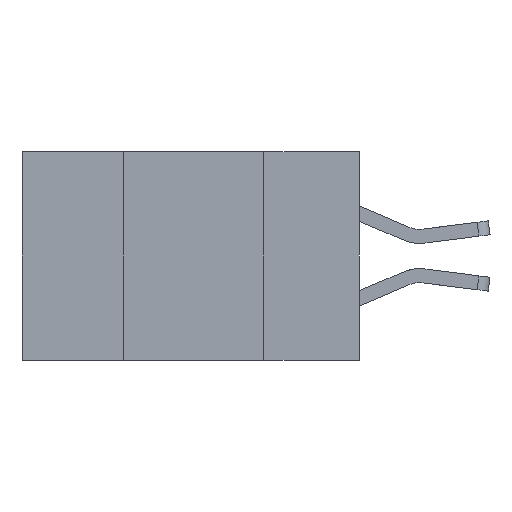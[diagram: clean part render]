
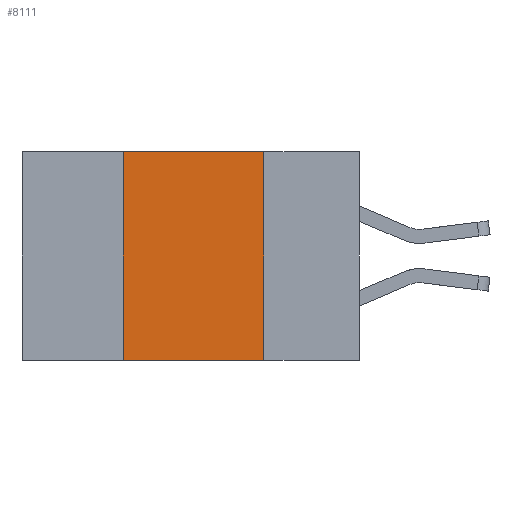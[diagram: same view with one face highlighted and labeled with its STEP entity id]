
A CAD part, left-side view. The second image highlights one B-rep face of the part: STEP entity #8111.
In plain terms, the highlighted planar face has unit normal (-1, 0, 0).
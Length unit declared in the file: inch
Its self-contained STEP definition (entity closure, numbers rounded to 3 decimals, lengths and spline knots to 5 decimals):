
#244 = CARTESIAN_POINT ( 'NONE',  ( 0., 0.42, 0. ) ) ;
#559 = CARTESIAN_POINT ( 'NONE',  ( 0., 0.17, 0. ) ) ;
#1182 = VERTEX_POINT ( 'NONE', #559 ) ;
#1582 = PLANE ( 'NONE',  #7429 ) ;
#2369 = VERTEX_POINT ( 'NONE', #5962 ) ;
#2441 = FACE_OUTER_BOUND ( 'NONE', #2443, .T. ) ;
#2443 = EDGE_LOOP ( 'NONE', ( #5814, #4598, #8984, #4454 ) ) ;
#2475 = DIRECTION ( 'NONE',  ( 0., 0., -1. ) ) ;
#2588 = CARTESIAN_POINT ( 'NONE',  ( 0., 0.6, -0.37 ) ) ;
#2659 = CARTESIAN_POINT ( 'NONE',  ( 0., 0.17, 0. ) ) ;
#3174 = DIRECTION ( 'NONE',  ( 1., 0., 0. ) ) ;
#3296 = VECTOR ( 'NONE', #6141, 39.37008 ) ;
#3353 = DIRECTION ( 'NONE',  ( 0., -1., 0. ) ) ;
#3984 = VECTOR ( 'NONE', #2475, 39.37008 ) ;
#4454 = ORIENTED_EDGE ( 'NONE', *, *, #8288, .T. ) ;
#4598 = ORIENTED_EDGE ( 'NONE', *, *, #5937, .F. ) ;
#4675 = LINE ( 'NONE', #8210, #8160 ) ;
#5229 = LINE ( 'NONE', #2588, #8455 ) ;
#5239 = LINE ( 'NONE', #6143, #3296 ) ;
#5747 = EDGE_CURVE ( 'NONE', #2369, #7401, #4675, .T. ) ;
#5814 = ORIENTED_EDGE ( 'NONE', *, *, #6689, .F. ) ;
#5937 = EDGE_CURVE ( 'NONE', #7401, #1182, #5239, .T. ) ;
#5962 = CARTESIAN_POINT ( 'NONE',  ( 0., 0.42, -0.37 ) ) ;
#6141 = DIRECTION ( 'NONE',  ( 0., -1., 0. ) ) ;
#6143 = CARTESIAN_POINT ( 'NONE',  ( 0., 0.6, 0. ) ) ;
#6538 = VERTEX_POINT ( 'NONE', #7768 ) ;
#6689 = EDGE_CURVE ( 'NONE', #1182, #6538, #7922, .T. ) ;
#7401 = VERTEX_POINT ( 'NONE', #244 ) ;
#7422 = CARTESIAN_POINT ( 'NONE',  ( 0., 0.6, 0. ) ) ;
#7429 = AXIS2_PLACEMENT_3D ( 'NONE', #7422, #3174, #8116 ) ;
#7768 = CARTESIAN_POINT ( 'NONE',  ( 0., 0.17, -0.37 ) ) ;
#7922 = LINE ( 'NONE', #2659, #3984 ) ;
#8111 = ADVANCED_FACE ( 'NONE', ( #2441 ), #1582, .F. ) ;
#8116 = DIRECTION ( 'NONE',  ( 0., 0., -1. ) ) ;
#8160 = VECTOR ( 'NONE', #8199, 39.37008 ) ;
#8199 = DIRECTION ( 'NONE',  ( 0., 0., 1. ) ) ;
#8210 = CARTESIAN_POINT ( 'NONE',  ( 0., 0.42, 0. ) ) ;
#8288 = EDGE_CURVE ( 'NONE', #2369, #6538, #5229, .T. ) ;
#8455 = VECTOR ( 'NONE', #3353, 39.37008 ) ;
#8984 = ORIENTED_EDGE ( 'NONE', *, *, #5747, .F. ) ;
